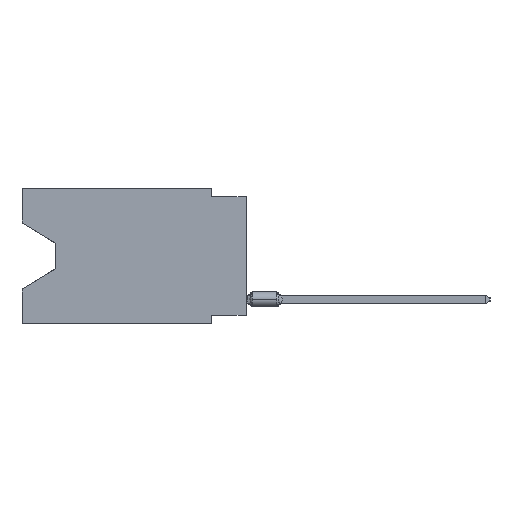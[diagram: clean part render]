
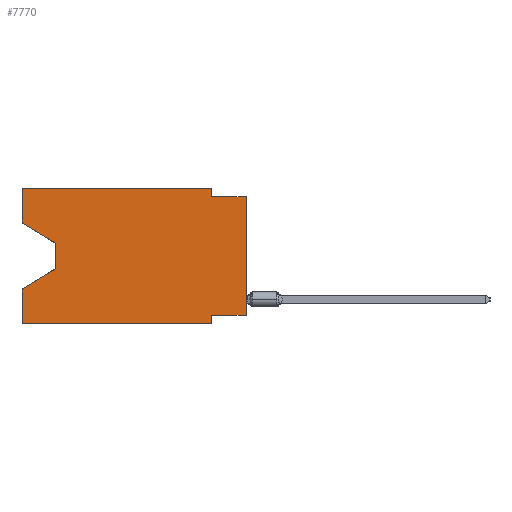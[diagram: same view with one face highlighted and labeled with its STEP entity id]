
A CAD part, left-side view. The second image highlights one B-rep face of the part: STEP entity #7770.
In plain terms, the highlighted planar face has unit normal (-1, 0, 0).
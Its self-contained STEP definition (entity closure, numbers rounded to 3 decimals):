
#105 = CARTESIAN_POINT ( 'NONE',  ( 0., 2.54, -0.635 ) ) ;
#332 = VECTOR ( 'NONE', #21115, 1000. ) ;
#517 = VERTEX_POINT ( 'NONE', #43615 ) ;
#1037 = CARTESIAN_POINT ( 'NONE',  ( 0., 16.383, 0. ) ) ;
#1543 = VECTOR ( 'NONE', #31784, 1000. ) ;
#1991 = CARTESIAN_POINT ( 'NONE',  ( 0., 0., -0.635 ) ) ;
#2338 = VERTEX_POINT ( 'NONE', #22823 ) ;
#2912 = VECTOR ( 'NONE', #49895, 1000. ) ;
#3891 = VECTOR ( 'NONE', #20166, 1000. ) ;
#4685 = PLANE ( 'NONE',  #45023 ) ;
#5574 = CARTESIAN_POINT ( 'NONE',  ( 0., 13.97, -5.893 ) ) ;
#6356 = DIRECTION ( 'NONE',  ( 0., 0., 1. ) ) ;
#7060 = EDGE_CURVE ( 'NONE', #55400, #517, #44041, .T. ) ;
#7373 = CARTESIAN_POINT ( 'NONE',  ( 0., 16.383, 0. ) ) ;
#7770 = ADVANCED_FACE ( 'NONE', ( #37958 ), #4685, .F. ) ;
#8717 = VERTEX_POINT ( 'NONE', #55708 ) ;
#8952 = DIRECTION ( 'NONE',  ( 0., 0., -1. ) ) ;
#9443 = ORIENTED_EDGE ( 'NONE', *, *, #61608, .T. ) ;
#10528 = EDGE_CURVE ( 'NONE', #8717, #14842, #56677, .T. ) ;
#11286 = LINE ( 'NONE', #16317, #2912 ) ;
#11406 = LINE ( 'NONE', #1991, #332 ) ;
#12064 = LINE ( 'NONE', #7373, #21253 ) ;
#12465 = EDGE_CURVE ( 'NONE', #17828, #37184, #12064, .T. ) ;
#12633 = CARTESIAN_POINT ( 'NONE',  ( 0., 13.97, -5.893 ) ) ;
#13202 = VECTOR ( 'NONE', #8952, 1000. ) ;
#13630 = EDGE_CURVE ( 'NONE', #2338, #61763, #16700, .T. ) ;
#13672 = CARTESIAN_POINT ( 'NONE',  ( 0., 13.97, -4.013 ) ) ;
#14256 = LINE ( 'NONE', #38428, #46367 ) ;
#14842 = VERTEX_POINT ( 'NONE', #5574 ) ;
#14857 = ORIENTED_EDGE ( 'NONE', *, *, #10528, .T. ) ;
#16317 = CARTESIAN_POINT ( 'NONE',  ( 0., 0., -9.271 ) ) ;
#16400 = LINE ( 'NONE', #39936, #60027 ) ;
#16512 = DIRECTION ( 'NONE',  ( 0., -0.855, -0.519 ) ) ;
#16700 = LINE ( 'NONE', #26430, #23373 ) ;
#16980 = DIRECTION ( 'NONE',  ( 0., -1., 0. ) ) ;
#17089 = DIRECTION ( 'NONE',  ( 0., 0., 1. ) ) ;
#17430 = CARTESIAN_POINT ( 'NONE',  ( 0., 16.383, -2.546 ) ) ;
#17440 = CARTESIAN_POINT ( 'NONE',  ( 0., 16.383, 0. ) ) ;
#17828 = VERTEX_POINT ( 'NONE', #24654 ) ;
#18031 = CARTESIAN_POINT ( 'NONE',  ( 0., 0., -0.635 ) ) ;
#18325 = EDGE_CURVE ( 'NONE', #49196, #55400, #16400, .T. ) ;
#18742 = EDGE_CURVE ( 'NONE', #2338, #30820, #11286, .T. ) ;
#18792 = DIRECTION ( 'NONE',  ( 0., 0., -1. ) ) ;
#19580 = VECTOR ( 'NONE', #56178, 1000. ) ;
#20166 = DIRECTION ( 'NONE',  ( 0., -1., 0. ) ) ;
#21115 = DIRECTION ( 'NONE',  ( 0., -1., 0. ) ) ;
#21253 = VECTOR ( 'NONE', #17089, 1000. ) ;
#21700 = DIRECTION ( 'NONE',  ( 0., 0., 1. ) ) ;
#22823 = CARTESIAN_POINT ( 'NONE',  ( 0., 0., -9.271 ) ) ;
#23324 = ORIENTED_EDGE ( 'NONE', *, *, #13630, .T. ) ;
#23373 = VECTOR ( 'NONE', #21700, 1000. ) ;
#24654 = CARTESIAN_POINT ( 'NONE',  ( 0., 16.383, -9.906 ) ) ;
#25578 = ORIENTED_EDGE ( 'NONE', *, *, #12465, .F. ) ;
#26430 = CARTESIAN_POINT ( 'NONE',  ( 0., 0., 0. ) ) ;
#30820 = VERTEX_POINT ( 'NONE', #32593 ) ;
#31096 = EDGE_CURVE ( 'NONE', #17828, #40198, #44918, .T. ) ;
#31784 = DIRECTION ( 'NONE',  ( 0., 0.855, -0.519 ) ) ;
#32593 = CARTESIAN_POINT ( 'NONE',  ( 0., 2.54, -9.271 ) ) ;
#33896 = ORIENTED_EDGE ( 'NONE', *, *, #35747, .F. ) ;
#35747 = EDGE_CURVE ( 'NONE', #30820, #40198, #14256, .T. ) ;
#37184 = VERTEX_POINT ( 'NONE', #57437 ) ;
#37958 = FACE_OUTER_BOUND ( 'NONE', #45341, .T. ) ;
#37966 = CARTESIAN_POINT ( 'NONE',  ( 0., 2.54, 0. ) ) ;
#38428 = CARTESIAN_POINT ( 'NONE',  ( 0., 2.54, -9.906 ) ) ;
#38676 = ORIENTED_EDGE ( 'NONE', *, *, #39126, .T. ) ;
#38763 = ORIENTED_EDGE ( 'NONE', *, *, #46323, .F. ) ;
#39126 = EDGE_CURVE ( 'NONE', #14842, #37184, #60375, .T. ) ;
#39936 = CARTESIAN_POINT ( 'NONE',  ( 0., 16.383, 0. ) ) ;
#40198 = VERTEX_POINT ( 'NONE', #44453 ) ;
#43402 = VECTOR ( 'NONE', #16512, 1000. ) ;
#43589 = VERTEX_POINT ( 'NONE', #105 ) ;
#43615 = CARTESIAN_POINT ( 'NONE',  ( 0., 2.54, 0. ) ) ;
#44041 = LINE ( 'NONE', #1037, #3891 ) ;
#44453 = CARTESIAN_POINT ( 'NONE',  ( 0., 2.54, -9.906 ) ) ;
#44893 = ORIENTED_EDGE ( 'NONE', *, *, #31096, .T. ) ;
#44918 = LINE ( 'NONE', #45861, #56556 ) ;
#45023 = AXIS2_PLACEMENT_3D ( 'NONE', #52393, #47679, #18792 ) ;
#45341 = EDGE_LOOP ( 'NONE', ( #9443, #14857, #38676, #25578, #44893, #33896, #46106, #23324, #60584, #38763, #61261, #52312 ) ) ;
#45861 = CARTESIAN_POINT ( 'NONE',  ( 0., 16.383, -9.906 ) ) ;
#46106 = ORIENTED_EDGE ( 'NONE', *, *, #18742, .F. ) ;
#46323 = EDGE_CURVE ( 'NONE', #517, #43589, #53783, .T. ) ;
#46367 = VECTOR ( 'NONE', #56963, 1000. ) ;
#47679 = DIRECTION ( 'NONE',  ( 1., 0., 0. ) ) ;
#49196 = VERTEX_POINT ( 'NONE', #55631 ) ;
#49895 = DIRECTION ( 'NONE',  ( 0., 1., 0. ) ) ;
#50708 = LINE ( 'NONE', #17430, #43402 ) ;
#52312 = ORIENTED_EDGE ( 'NONE', *, *, #18325, .F. ) ;
#52393 = CARTESIAN_POINT ( 'NONE',  ( 0., 16.383, 0. ) ) ;
#53783 = LINE ( 'NONE', #37966, #19580 ) ;
#55400 = VERTEX_POINT ( 'NONE', #17440 ) ;
#55631 = CARTESIAN_POINT ( 'NONE',  ( 0., 16.383, -2.546 ) ) ;
#55708 = CARTESIAN_POINT ( 'NONE',  ( 0., 13.97, -4.013 ) ) ;
#56178 = DIRECTION ( 'NONE',  ( 0., 0., -1. ) ) ;
#56556 = VECTOR ( 'NONE', #16980, 1000. ) ;
#56677 = LINE ( 'NONE', #13672, #13202 ) ;
#56963 = DIRECTION ( 'NONE',  ( 0., 0., -1. ) ) ;
#57437 = CARTESIAN_POINT ( 'NONE',  ( 0., 16.383, -7.36 ) ) ;
#60027 = VECTOR ( 'NONE', #6356, 1000. ) ;
#60375 = LINE ( 'NONE', #12633, #1543 ) ;
#60584 = ORIENTED_EDGE ( 'NONE', *, *, #62000, .F. ) ;
#61261 = ORIENTED_EDGE ( 'NONE', *, *, #7060, .F. ) ;
#61608 = EDGE_CURVE ( 'NONE', #49196, #8717, #50708, .T. ) ;
#61763 = VERTEX_POINT ( 'NONE', #18031 ) ;
#62000 = EDGE_CURVE ( 'NONE', #43589, #61763, #11406, .T. ) ;
